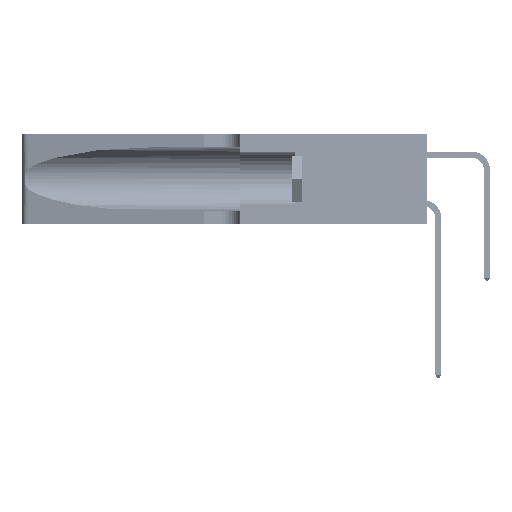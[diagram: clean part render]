
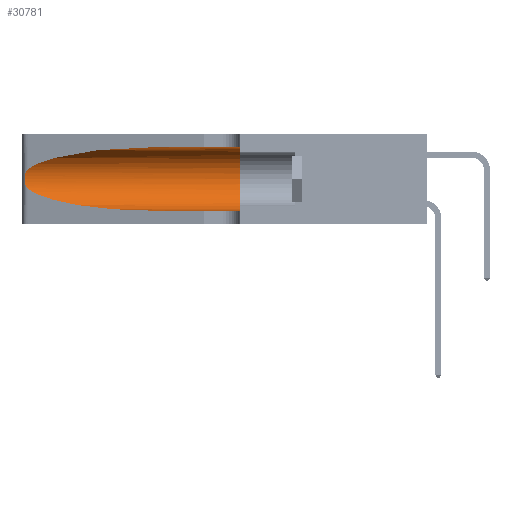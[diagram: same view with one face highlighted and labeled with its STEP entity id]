
A CAD part, left-side view. The second image highlights one B-rep face of the part: STEP entity #30781.
In plain terms, the highlighted cylindrical face has radius 3.308 mm (diameter 6.617 mm), a partial arc.
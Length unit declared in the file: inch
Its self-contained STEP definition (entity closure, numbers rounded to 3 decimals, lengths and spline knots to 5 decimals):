
#328 = CARTESIAN_POINT ( 'NONE',  ( 0.25639, 1.23186, 0.15144 ) ) ;
#666 = CARTESIAN_POINT ( 'NONE',  ( 0.1305, 0.72297, 0.31525 ) ) ;
#1266 = EDGE_LOOP ( 'NONE', ( #1566, #36745, #18662, #43597, #36803, #35489 ) ) ;
#1566 = ORIENTED_EDGE ( 'NONE', *, *, #32755, .T. ) ;
#3230 = CARTESIAN_POINT ( 'NONE',  ( 0.1305, 0.35, 0.31525 ) ) ;
#4598 = CARTESIAN_POINT ( 'NONE',  ( 0.25487, 1.22718, 0.14631 ) ) ;
#5531 = B_SPLINE_CURVE_WITH_KNOTS ( 'NONE', 3,
 ( #45884, #21070, #8656, #37777, #12852, #41939, #17047, #46060, #21245, #50169, #25431, #328, #29597, #4598 ),
 .UNSPECIFIED., .F., .F.,
 ( 4, 2, 2, 2, 2, 2, 4 ),
 ( 0., 0.00027, 0.00053, 0.00107, 0.0016, 0.00187, 0.00214 ),
 .UNSPECIFIED. ) ;
#6417 = CARTESIAN_POINT ( 'NONE',  ( 0.1305, 0.72297, 0.05475 ) ) ;
#6980 = CARTESIAN_POINT ( 'NONE',  ( 0.1305, 0.72297, 0.31525 ) ) ;
#7871 = CARTESIAN_POINT ( 'NONE',  ( 0.25487, 1.22718, 0.22369 ) ) ;
#8656 = CARTESIAN_POINT ( 'NONE',  ( 0.25639, 1.23184, 0.21858 ) ) ;
#9197 = AXIS2_PLACEMENT_3D ( 'NONE', #15735, #19945, #24122 ) ;
#9232 = CARTESIAN_POINT ( 'NONE',  ( 0.1305, 1.61858, 0.05475 ) ) ;
#9412 = DIRECTION ( 'NONE',  ( 0., -1., 0. ) ) ;
#11182 = CARTESIAN_POINT ( 'NONE',  ( 0.25487, 1.22718, 0.22369 ) ) ;
#12852 = CARTESIAN_POINT ( 'NONE',  ( 0.25854, 1.2359, 0.20912 ) ) ;
#14893 = CARTESIAN_POINT ( 'NONE',  ( 0.1305, 0.72297, 0.05475 ) ) ;
#15350 = EDGE_CURVE ( 'NONE', #32835, #48712, #47290, .T. ) ;
#15735 = CARTESIAN_POINT ( 'NONE',  ( 0.1305, 1.61858, 0.185 ) ) ;
#17047 = CARTESIAN_POINT ( 'NONE',  ( 0.26075, 1.23896, 0.19203 ) ) ;
#17875 = FACE_OUTER_BOUND ( 'NONE', #1266, .T. ) ;
#18662 = ORIENTED_EDGE ( 'NONE', *, *, #50402, .T. ) ;
#19271 =( BOUNDED_CURVE ( )  B_SPLINE_CURVE ( 3, ( #6980, #19400, #52456, #11182 ),
 .UNSPECIFIED., .F., .F. ) 
 B_SPLINE_CURVE_WITH_KNOTS ( ( 4, 4 ),
 ( 1.5708, 2.84003 ),
 .UNSPECIFIED. ) 
 CURVE ( )  GEOMETRIC_REPRESENTATION_ITEM ( )  RATIONAL_B_SPLINE_CURVE ( ( 1., 0.87, 0.87, 1. ) ) 
 REPRESENTATION_ITEM ( '' )  );
#19400 = CARTESIAN_POINT ( 'NONE',  ( 0.18966, 0.96281, 0.31525 ) ) ;
#19945 = DIRECTION ( 'NONE',  ( 0., -1., 0. ) ) ;
#21070 = CARTESIAN_POINT ( 'NONE',  ( 0.25555, 1.22994, 0.2215 ) ) ;
#21245 = CARTESIAN_POINT ( 'NONE',  ( 0.26017, 1.23833, 0.17102 ) ) ;
#22619 = CARTESIAN_POINT ( 'NONE',  ( 0.1305, 0.35, 0.185 ) ) ;
#24122 = DIRECTION ( 'NONE',  ( 0., 0., -1. ) ) ;
#24927 =( BOUNDED_CURVE ( )  B_SPLINE_CURVE ( 3, ( #43694, #31213, #31398, #6417 ),
 .UNSPECIFIED., .F., .F. ) 
 B_SPLINE_CURVE_WITH_KNOTS ( ( 4, 4 ),
 ( 3.44316, 4.71239 ),
 .UNSPECIFIED. ) 
 CURVE ( )  GEOMETRIC_REPRESENTATION_ITEM ( )  RATIONAL_B_SPLINE_CURVE ( ( 1., 0.87, 0.87, 1. ) ) 
 REPRESENTATION_ITEM ( '' )  );
#25431 = CARTESIAN_POINT ( 'NONE',  ( 0.25789, 1.23486, 0.15765 ) ) ;
#26803 = DIRECTION ( 'NONE',  ( 0., 0., 1. ) ) ;
#28036 = VERTEX_POINT ( 'NONE', #33355 ) ;
#29597 = CARTESIAN_POINT ( 'NONE',  ( 0.25555, 1.22993, 0.14849 ) ) ;
#30294 = EDGE_CURVE ( 'NONE', #34396, #48712, #52213, .T. ) ;
#30781 = ADVANCED_FACE ( 'NONE', ( #17875 ), #32877, .F. ) ;
#31213 = CARTESIAN_POINT ( 'NONE',  ( 0.2373, 1.15595, 0.08982 ) ) ;
#31398 = CARTESIAN_POINT ( 'NONE',  ( 0.18966, 0.96281, 0.05475 ) ) ;
#32749 = CARTESIAN_POINT ( 'NONE',  ( 0.1305, 1.61858, 0.31525 ) ) ;
#32755 = EDGE_CURVE ( 'NONE', #46709, #45750, #19271, .T. ) ;
#32835 = VERTEX_POINT ( 'NONE', #3230 ) ;
#32877 = CYLINDRICAL_SURFACE ( 'NONE', #9197, 0.13025 ) ;
#33355 = CARTESIAN_POINT ( 'NONE',  ( 0.25487, 1.22718, 0.14631 ) ) ;
#34396 = VERTEX_POINT ( 'NONE', #14893 ) ;
#34609 = EDGE_CURVE ( 'NONE', #46709, #32835, #50681, .T. ) ;
#35489 = ORIENTED_EDGE ( 'NONE', *, *, #34609, .F. ) ;
#36745 = ORIENTED_EDGE ( 'NONE', *, *, #52026, .T. ) ;
#36803 = ORIENTED_EDGE ( 'NONE', *, *, #15350, .F. ) ;
#36910 = DIRECTION ( 'NONE',  ( 0., -1., 0. ) ) ;
#37567 = CARTESIAN_POINT ( 'NONE',  ( 0.1305, 0.35, 0.05475 ) ) ;
#37777 = CARTESIAN_POINT ( 'NONE',  ( 0.25787, 1.23484, 0.2124 ) ) ;
#38385 = AXIS2_PLACEMENT_3D ( 'NONE', #22619, #51528, #26803 ) ;
#39757 = VECTOR ( 'NONE', #36910, 39.37008 ) ;
#41939 = CARTESIAN_POINT ( 'NONE',  ( 0.26018, 1.23835, 0.19895 ) ) ;
#43597 = ORIENTED_EDGE ( 'NONE', *, *, #30294, .T. ) ;
#43694 = CARTESIAN_POINT ( 'NONE',  ( 0.25487, 1.22718, 0.14631 ) ) ;
#45750 = VERTEX_POINT ( 'NONE', #7871 ) ;
#45884 = CARTESIAN_POINT ( 'NONE',  ( 0.25487, 1.22718, 0.22369 ) ) ;
#46060 = CARTESIAN_POINT ( 'NONE',  ( 0.26075, 1.23896, 0.178 ) ) ;
#46709 = VERTEX_POINT ( 'NONE', #666 ) ;
#47290 = CIRCLE ( 'NONE', #38385, 0.13025 ) ;
#48712 = VERTEX_POINT ( 'NONE', #37567 ) ;
#50169 = CARTESIAN_POINT ( 'NONE',  ( 0.25856, 1.23593, 0.16098 ) ) ;
#50402 = EDGE_CURVE ( 'NONE', #28036, #34396, #24927, .T. ) ;
#50681 = LINE ( 'NONE', #32749, #39757 ) ;
#50934 = VECTOR ( 'NONE', #9412, 39.37008 ) ;
#51528 = DIRECTION ( 'NONE',  ( 0., 1., 0. ) ) ;
#52026 = EDGE_CURVE ( 'NONE', #45750, #28036, #5531, .T. ) ;
#52213 = LINE ( 'NONE', #9232, #50934 ) ;
#52456 = CARTESIAN_POINT ( 'NONE',  ( 0.2373, 1.15595, 0.28018 ) ) ;
